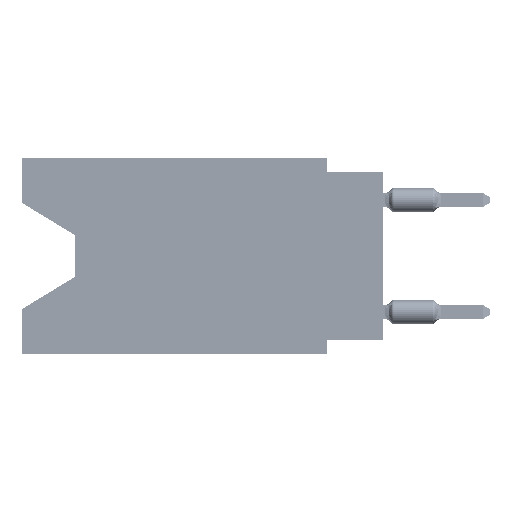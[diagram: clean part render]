
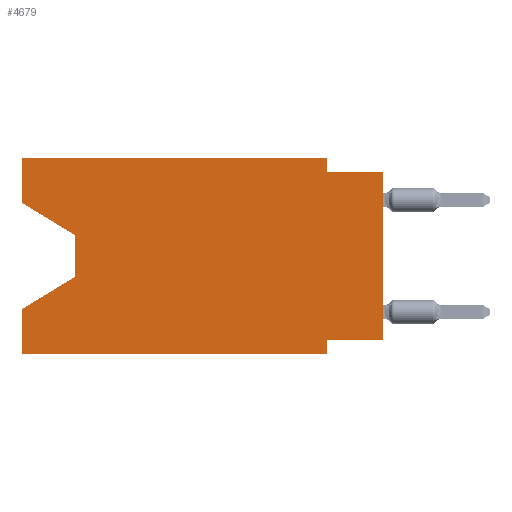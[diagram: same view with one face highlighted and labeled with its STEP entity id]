
A CAD part, left-side view. The second image highlights one B-rep face of the part: STEP entity #4679.
In plain terms, the highlighted planar face has unit normal (-1, 0, 0).
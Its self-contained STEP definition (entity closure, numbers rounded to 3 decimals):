
#323 = LINE ( 'NONE', #57227, #16671 ) ;
#2468 = ORIENTED_EDGE ( 'NONE', *, *, #70584, .F. ) ;
#2714 = LINE ( 'NONE', #53030, #6069 ) ;
#2729 = VERTEX_POINT ( 'NONE', #68621 ) ;
#3891 = DIRECTION ( 'NONE',  ( 0., 0., 1. ) ) ;
#4393 = VECTOR ( 'NONE', #22569, 1000. ) ;
#4421 = VERTEX_POINT ( 'NONE', #61550 ) ;
#4679 = ADVANCED_FACE ( 'NONE', ( #43482 ), #70318, .F. ) ;
#5368 = DIRECTION ( 'NONE',  ( 0., -0.855, -0.519 ) ) ;
#5849 = ORIENTED_EDGE ( 'NONE', *, *, #41071, .F. ) ;
#5890 = EDGE_CURVE ( 'NONE', #2729, #4421, #64104, .T. ) ;
#6069 = VECTOR ( 'NONE', #29886, 1000. ) ;
#6555 = ORIENTED_EDGE ( 'NONE', *, *, #52157, .T. ) ;
#7214 = CARTESIAN_POINT ( 'NONE',  ( 0., 13.97, -3.505 ) ) ;
#8997 = CARTESIAN_POINT ( 'NONE',  ( 0., 0., -8.255 ) ) ;
#10796 = CARTESIAN_POINT ( 'NONE',  ( 0., 16.383, 0. ) ) ;
#11615 = LINE ( 'NONE', #17493, #40525 ) ;
#12264 = CARTESIAN_POINT ( 'NONE',  ( 0., 16.383, -8.89 ) ) ;
#13149 = CARTESIAN_POINT ( 'NONE',  ( 0., 0., -0.635 ) ) ;
#13773 = LINE ( 'NONE', #41322, #55553 ) ;
#14518 = LINE ( 'NONE', #8997, #21375 ) ;
#15055 = VERTEX_POINT ( 'NONE', #31977 ) ;
#15353 = VERTEX_POINT ( 'NONE', #23499 ) ;
#15844 = EDGE_CURVE ( 'NONE', #59443, #15055, #14518, .T. ) ;
#16671 = VECTOR ( 'NONE', #45846, 1000. ) ;
#17493 = CARTESIAN_POINT ( 'NONE',  ( 0., 0., -0.635 ) ) ;
#18050 = ORIENTED_EDGE ( 'NONE', *, *, #51132, .F. ) ;
#18167 = EDGE_LOOP ( 'NONE', ( #6555, #27431, #48501, #68466, #61009, #52600, #29796, #21873, #5849, #18050, #27264, #2468 ) ) ;
#19937 = VERTEX_POINT ( 'NONE', #7214 ) ;
#20356 = LINE ( 'NONE', #37223, #40863 ) ;
#20496 = VERTEX_POINT ( 'NONE', #12264 ) ;
#20717 = DIRECTION ( 'NONE',  ( 0., 0., -1. ) ) ;
#21375 = VECTOR ( 'NONE', #64115, 1000. ) ;
#21873 = ORIENTED_EDGE ( 'NONE', *, *, #60153, .T. ) ;
#22569 = DIRECTION ( 'NONE',  ( 0., 0., 1. ) ) ;
#22641 = CARTESIAN_POINT ( 'NONE',  ( 0., 16.383, -2.038 ) ) ;
#23291 = LINE ( 'NONE', #10796, #4393 ) ;
#23499 = CARTESIAN_POINT ( 'NONE',  ( 0., 2.54, 0. ) ) ;
#23712 = EDGE_CURVE ( 'NONE', #20496, #4421, #25580, .T. ) ;
#23848 = VERTEX_POINT ( 'NONE', #67389 ) ;
#25398 = EDGE_CURVE ( 'NONE', #42764, #15353, #20356, .T. ) ;
#25580 = LINE ( 'NONE', #26647, #67839 ) ;
#26647 = CARTESIAN_POINT ( 'NONE',  ( 0., 16.383, 0. ) ) ;
#27264 = ORIENTED_EDGE ( 'NONE', *, *, #25398, .F. ) ;
#27429 = DIRECTION ( 'NONE',  ( 0., -1., 0. ) ) ;
#27431 = ORIENTED_EDGE ( 'NONE', *, *, #39040, .T. ) ;
#28535 = VECTOR ( 'NONE', #5368, 1000. ) ;
#29796 = ORIENTED_EDGE ( 'NONE', *, *, #15844, .F. ) ;
#29886 = DIRECTION ( 'NONE',  ( 0., -1., 0. ) ) ;
#30218 = VECTOR ( 'NONE', #20717, 1000. ) ;
#31977 = CARTESIAN_POINT ( 'NONE',  ( 0., 2.54, -8.255 ) ) ;
#32458 = DIRECTION ( 'NONE',  ( 0., 0., -1. ) ) ;
#33949 = CARTESIAN_POINT ( 'NONE',  ( 0., 16.383, 0. ) ) ;
#35814 = DIRECTION ( 'NONE',  ( 0., 0.855, -0.519 ) ) ;
#36342 = CARTESIAN_POINT ( 'NONE',  ( 0., 2.54, -8.89 ) ) ;
#37223 = CARTESIAN_POINT ( 'NONE',  ( 0., 16.383, 0. ) ) ;
#38657 = LINE ( 'NONE', #44546, #30218 ) ;
#39040 = EDGE_CURVE ( 'NONE', #19937, #2729, #38657, .T. ) ;
#40448 = VERTEX_POINT ( 'NONE', #41518 ) ;
#40525 = VECTOR ( 'NONE', #27429, 1000. ) ;
#40863 = VECTOR ( 'NONE', #59635, 1000. ) ;
#41041 = VECTOR ( 'NONE', #35814, 1000. ) ;
#41071 = EDGE_CURVE ( 'NONE', #55248, #56177, #11615, .T. ) ;
#41322 = CARTESIAN_POINT ( 'NONE',  ( 0., 0., 0. ) ) ;
#41518 = CARTESIAN_POINT ( 'NONE',  ( 0., 2.54, -8.89 ) ) ;
#42764 = VERTEX_POINT ( 'NONE', #33949 ) ;
#43482 = FACE_OUTER_BOUND ( 'NONE', #18167, .T. ) ;
#44546 = CARTESIAN_POINT ( 'NONE',  ( 0., 13.97, -3.505 ) ) ;
#45846 = DIRECTION ( 'NONE',  ( 0., 0., -1. ) ) ;
#47376 = LINE ( 'NONE', #36342, #57250 ) ;
#48501 = ORIENTED_EDGE ( 'NONE', *, *, #5890, .T. ) ;
#51132 = EDGE_CURVE ( 'NONE', #15353, #55248, #323, .T. ) ;
#51983 = DIRECTION ( 'NONE',  ( 0., 0., 1. ) ) ;
#52157 = EDGE_CURVE ( 'NONE', #23848, #19937, #53620, .T. ) ;
#52252 = CARTESIAN_POINT ( 'NONE',  ( 0., 0., -8.255 ) ) ;
#52600 = ORIENTED_EDGE ( 'NONE', *, *, #71058, .F. ) ;
#53030 = CARTESIAN_POINT ( 'NONE',  ( 0., 16.383, -8.89 ) ) ;
#53620 = LINE ( 'NONE', #22641, #28535 ) ;
#54154 = DIRECTION ( 'NONE',  ( 1., 0., 0. ) ) ;
#55248 = VERTEX_POINT ( 'NONE', #55584 ) ;
#55553 = VECTOR ( 'NONE', #51983, 1000. ) ;
#55584 = CARTESIAN_POINT ( 'NONE',  ( 0., 2.54, -0.635 ) ) ;
#56177 = VERTEX_POINT ( 'NONE', #13149 ) ;
#57227 = CARTESIAN_POINT ( 'NONE',  ( 0., 2.54, 0. ) ) ;
#57250 = VECTOR ( 'NONE', #58753, 1000. ) ;
#58151 = EDGE_CURVE ( 'NONE', #20496, #40448, #2714, .T. ) ;
#58753 = DIRECTION ( 'NONE',  ( 0., 0., -1. ) ) ;
#59443 = VERTEX_POINT ( 'NONE', #52252 ) ;
#59635 = DIRECTION ( 'NONE',  ( 0., -1., 0. ) ) ;
#60153 = EDGE_CURVE ( 'NONE', #59443, #56177, #13773, .T. ) ;
#61009 = ORIENTED_EDGE ( 'NONE', *, *, #58151, .T. ) ;
#61550 = CARTESIAN_POINT ( 'NONE',  ( 0., 16.383, -6.852 ) ) ;
#63011 = CARTESIAN_POINT ( 'NONE',  ( 0., 13.97, -5.385 ) ) ;
#64104 = LINE ( 'NONE', #63011, #41041 ) ;
#64115 = DIRECTION ( 'NONE',  ( 0., 1., 0. ) ) ;
#65177 = CARTESIAN_POINT ( 'NONE',  ( 0., 16.383, 0. ) ) ;
#67389 = CARTESIAN_POINT ( 'NONE',  ( 0., 16.383, -2.038 ) ) ;
#67839 = VECTOR ( 'NONE', #3891, 1000. ) ;
#67867 = AXIS2_PLACEMENT_3D ( 'NONE', #65177, #54154, #32458 ) ;
#68466 = ORIENTED_EDGE ( 'NONE', *, *, #23712, .F. ) ;
#68621 = CARTESIAN_POINT ( 'NONE',  ( 0., 13.97, -5.385 ) ) ;
#70318 = PLANE ( 'NONE',  #67867 ) ;
#70584 = EDGE_CURVE ( 'NONE', #23848, #42764, #23291, .T. ) ;
#71058 = EDGE_CURVE ( 'NONE', #15055, #40448, #47376, .T. ) ;
